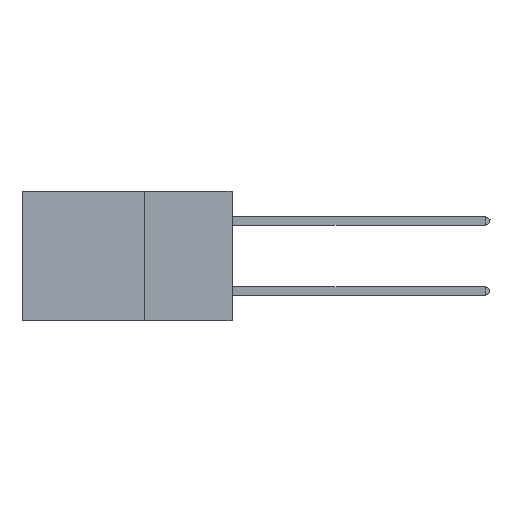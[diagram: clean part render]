
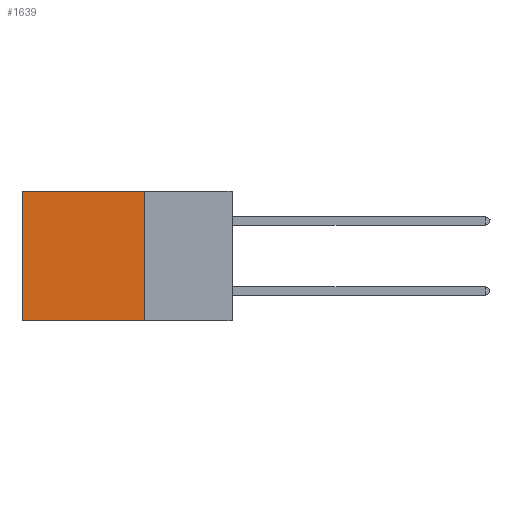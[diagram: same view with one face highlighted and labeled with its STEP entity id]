
A CAD part, left-side view. The second image highlights one B-rep face of the part: STEP entity #1639.
In plain terms, the highlighted planar face has unit normal (-1, 0, 0).
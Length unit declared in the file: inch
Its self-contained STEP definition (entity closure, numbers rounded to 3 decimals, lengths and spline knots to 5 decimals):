
#1089 = VECTOR ( 'NONE', #2145, 39.37008 ) ;
#1639 = ADVANCED_FACE ( 'NONE', ( #20281 ), #33933, .F. ) ;
#1696 = LINE ( 'NONE', #22544, #1089 ) ;
#2145 = DIRECTION ( 'NONE',  ( 0., 1., 0. ) ) ;
#5236 = VECTOR ( 'NONE', #28113, 39.37008 ) ;
#5847 = EDGE_CURVE ( 'NONE', #31501, #39751, #13566, .T. ) ;
#5959 = LINE ( 'NONE', #37524, #19259 ) ;
#12476 = ORIENTED_EDGE ( 'NONE', *, *, #43499, .T. ) ;
#13566 = LINE ( 'NONE', #17372, #5236 ) ;
#14342 = ORIENTED_EDGE ( 'NONE', *, *, #30038, .T. ) ;
#14594 = EDGE_CURVE ( 'NONE', #39751, #39914, #1696, .T. ) ;
#16284 = DIRECTION ( 'NONE',  ( 0., 0., -1. ) ) ;
#17372 = CARTESIAN_POINT ( 'NONE',  ( 0.2875, 0.25, 0. ) ) ;
#17813 = LINE ( 'NONE', #24543, #40216 ) ;
#18260 = DIRECTION ( 'NONE',  ( 0., 1., 0. ) ) ;
#19259 = VECTOR ( 'NONE', #16284, 39.37008 ) ;
#20281 = FACE_OUTER_BOUND ( 'NONE', #38374, .T. ) ;
#20552 = VERTEX_POINT ( 'NONE', #43101 ) ;
#22544 = CARTESIAN_POINT ( 'NONE',  ( 0.2875, 0.25, -0.37 ) ) ;
#22698 = CARTESIAN_POINT ( 'NONE',  ( 0.2875, 0.25, 0. ) ) ;
#23235 = CARTESIAN_POINT ( 'NONE',  ( 0.2875, 0.6, -0.37 ) ) ;
#24169 = ORIENTED_EDGE ( 'NONE', *, *, #14594, .F. ) ;
#24543 = CARTESIAN_POINT ( 'NONE',  ( 0.2875, 0.25, 0. ) ) ;
#27803 = ORIENTED_EDGE ( 'NONE', *, *, #5847, .F. ) ;
#28113 = DIRECTION ( 'NONE',  ( 0., 0., -1. ) ) ;
#30038 = EDGE_CURVE ( 'NONE', #31501, #20552, #17813, .T. ) ;
#30136 = CARTESIAN_POINT ( 'NONE',  ( 0.2875, 0.25, 0. ) ) ;
#31501 = VERTEX_POINT ( 'NONE', #22698 ) ;
#33933 = PLANE ( 'NONE',  #41225 ) ;
#37524 = CARTESIAN_POINT ( 'NONE',  ( 0.2875, 0.6, 0. ) ) ;
#38374 = EDGE_LOOP ( 'NONE', ( #12476, #24169, #27803, #14342 ) ) ;
#39751 = VERTEX_POINT ( 'NONE', #42952 ) ;
#39914 = VERTEX_POINT ( 'NONE', #23235 ) ;
#40216 = VECTOR ( 'NONE', #18260, 39.37008 ) ;
#41049 = DIRECTION ( 'NONE',  ( 0., 0., -1. ) ) ;
#41225 = AXIS2_PLACEMENT_3D ( 'NONE', #30136, #43818, #41049 ) ;
#42952 = CARTESIAN_POINT ( 'NONE',  ( 0.2875, 0.25, -0.37 ) ) ;
#43101 = CARTESIAN_POINT ( 'NONE',  ( 0.2875, 0.6, 0. ) ) ;
#43499 = EDGE_CURVE ( 'NONE', #20552, #39914, #5959, .T. ) ;
#43818 = DIRECTION ( 'NONE',  ( 1., 0., 0. ) ) ;
